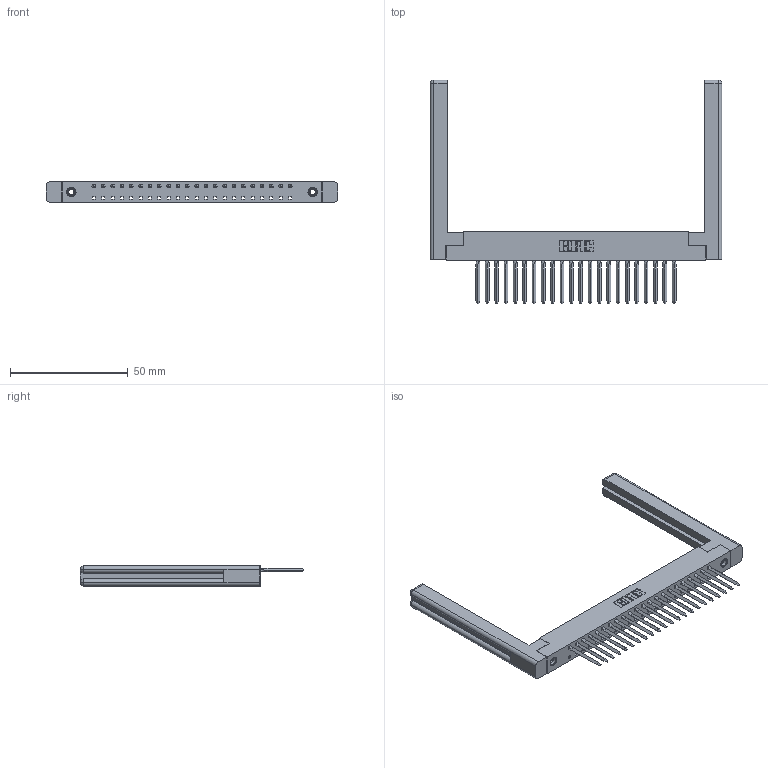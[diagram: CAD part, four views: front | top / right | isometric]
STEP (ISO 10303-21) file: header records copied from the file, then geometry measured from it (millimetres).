
FILE_DESCRIPTION (( 'STEP AP203' ), '1' );
FILE_NAME ('338-022-541-168.STEP', '2020-03-24T17:48:41', ( '' ), ( '' ), 'SwSTEP 2.0', 'SolidWorks 2016', '' );
FILE_SCHEMA (( 'CONFIG_CONTROL_DESIGN' ));
Length unit declared in the file: inch
Products named in the file (5): 338-290-001_541; 345-250-001_345-250-001-102; 338-210-001_338-210-022-004; 307-220-058; 338-022-541-168
Assembly tree (27 placements, depth 2):
  338-022-541-168
    338-210-001_338-210-022-004
    338-290-001_541  x22
    345-250-001_345-250-001-102  x2
    307-220-058  x2
Bounding box: 123.8 x 94.87 x 8.71 mm (x, y, z)
Volume: 16289.7 mm3; surface area: 19084.8 mm2
Topology: 27 solids, 27 shells, 2282 faces, 6259 edges, 3998 vertices
Faces by surface type: plane 1564, cylinder 606, bspline 88, cone 12, torus 12
Entity records: 46909 total; most frequent: CARTESIAN_POINT 9373, ORIENTED_EDGE 7874, DIRECTION 7372, EDGE_CURVE 3937, LINE 2926, VECTOR 2926, VERTEX_POINT 2554, AXIS2_PLACEMENT_3D 2223
